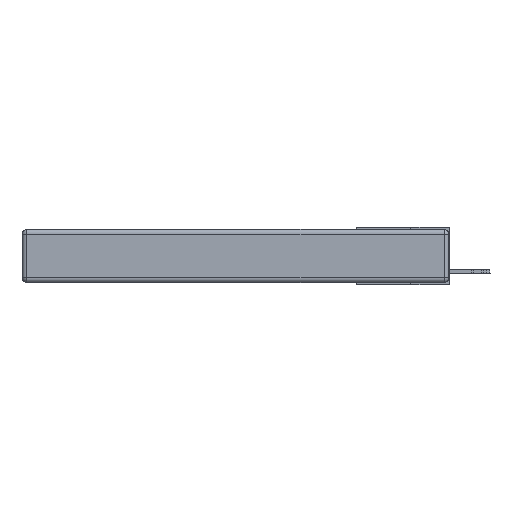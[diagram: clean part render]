
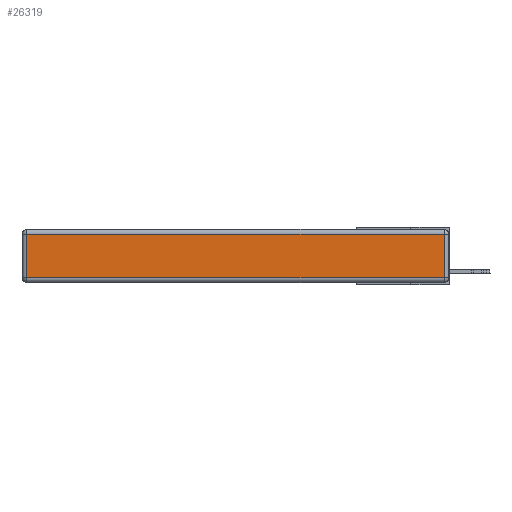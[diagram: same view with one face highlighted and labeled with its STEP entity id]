
A CAD part, left-side view. The second image highlights one B-rep face of the part: STEP entity #26319.
In plain terms, the highlighted planar face has unit normal (-1, 0, 0).
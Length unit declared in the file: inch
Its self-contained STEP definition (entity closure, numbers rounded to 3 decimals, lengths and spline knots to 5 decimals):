
#58 = CARTESIAN_POINT ( 'NONE',  ( 0., 2.72, -0.343 ) ) ;
#402 = VECTOR ( 'NONE', #4813, 39.37008 ) ;
#494 = LINE ( 'NONE', #13222, #9552 ) ;
#766 = DIRECTION ( 'NONE',  ( 0., -1., 0. ) ) ;
#904 = FACE_OUTER_BOUND ( 'NONE', #18187, .T. ) ;
#1703 = AXIS2_PLACEMENT_3D ( 'NONE', #2768, #27477, #18487 ) ;
#2768 = CARTESIAN_POINT ( 'NONE',  ( 0., 0., -0.343 ) ) ;
#3785 = VERTEX_POINT ( 'NONE', #26923 ) ;
#4208 = DIRECTION ( 'NONE',  ( 0., 1., 0. ) ) ;
#4258 = ORIENTED_EDGE ( 'NONE', *, *, #12696, .T. ) ;
#4813 = DIRECTION ( 'NONE',  ( 0., 0., -1. ) ) ;
#5417 = VERTEX_POINT ( 'NONE', #20056 ) ;
#5845 = EDGE_CURVE ( 'NONE', #12262, #21144, #494, .T. ) ;
#6321 = LINE ( 'NONE', #58, #402 ) ;
#6838 = VECTOR ( 'NONE', #8703, 39.37008 ) ;
#7536 = PLANE ( 'NONE',  #1703 ) ;
#8703 = DIRECTION ( 'NONE',  ( 0., 0., 1. ) ) ;
#9552 = VECTOR ( 'NONE', #4208, 39.37008 ) ;
#10986 = VECTOR ( 'NONE', #766, 39.37008 ) ;
#11216 = CARTESIAN_POINT ( 'NONE',  ( 0., 2.72, -0.03 ) ) ;
#11846 = ORIENTED_EDGE ( 'NONE', *, *, #5845, .T. ) ;
#12262 = VERTEX_POINT ( 'NONE', #23753 ) ;
#12696 = EDGE_CURVE ( 'NONE', #21144, #5417, #6321, .T. ) ;
#13222 = CARTESIAN_POINT ( 'NONE',  ( 0., 2.75, -0.03 ) ) ;
#14008 = CARTESIAN_POINT ( 'NONE',  ( 0., 0., -0.313 ) ) ;
#14686 = EDGE_CURVE ( 'NONE', #5417, #3785, #22954, .T. ) ;
#16648 = ORIENTED_EDGE ( 'NONE', *, *, #21629, .T. ) ;
#17655 = ORIENTED_EDGE ( 'NONE', *, *, #14686, .T. ) ;
#18187 = EDGE_LOOP ( 'NONE', ( #17655, #16648, #11846, #4258 ) ) ;
#18487 = DIRECTION ( 'NONE',  ( 0., 0., 1. ) ) ;
#20056 = CARTESIAN_POINT ( 'NONE',  ( 0., 2.72, -0.313 ) ) ;
#21144 = VERTEX_POINT ( 'NONE', #11216 ) ;
#21629 = EDGE_CURVE ( 'NONE', #3785, #12262, #24515, .T. ) ;
#22276 = CARTESIAN_POINT ( 'NONE',  ( 0., 0.03, -0.343 ) ) ;
#22954 = LINE ( 'NONE', #14008, #10986 ) ;
#23753 = CARTESIAN_POINT ( 'NONE',  ( 0., 0.03, -0.03 ) ) ;
#24515 = LINE ( 'NONE', #22276, #6838 ) ;
#26319 = ADVANCED_FACE ( 'NONE', ( #904 ), #7536, .T. ) ;
#26923 = CARTESIAN_POINT ( 'NONE',  ( 0., 0.03, -0.313 ) ) ;
#27477 = DIRECTION ( 'NONE',  ( -1., 0., 0. ) ) ;
